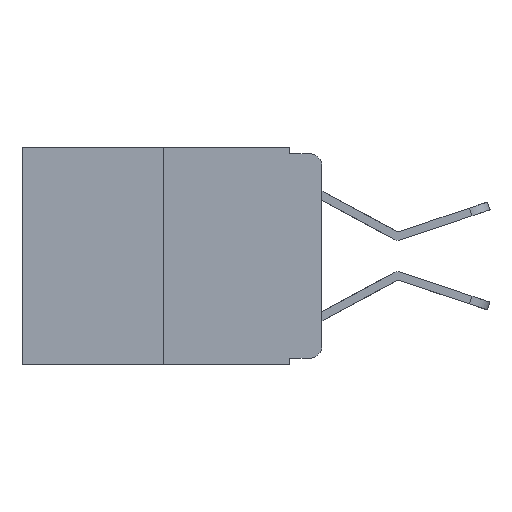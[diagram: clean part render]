
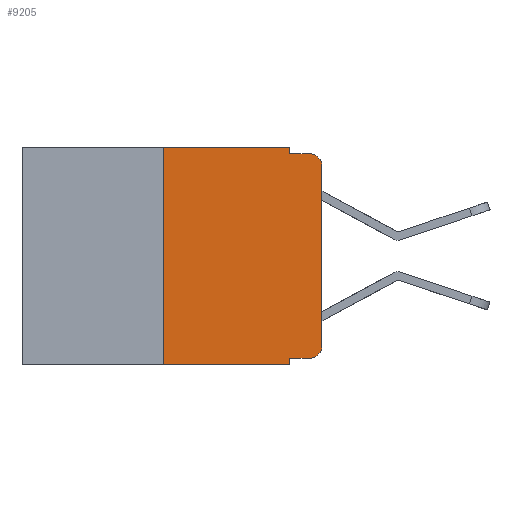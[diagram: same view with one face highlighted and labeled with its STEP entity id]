
A CAD part, left-side view. The second image highlights one B-rep face of the part: STEP entity #9205.
In plain terms, the highlighted planar face has unit normal (-1, 0, 0).
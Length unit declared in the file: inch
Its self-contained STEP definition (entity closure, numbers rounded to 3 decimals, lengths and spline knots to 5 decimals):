
#438 = CARTESIAN_POINT ( 'NONE',  ( 0., 0.051, -0.343 ) ) ;
#511 = DIRECTION ( 'NONE',  ( 0., 0., 1. ) ) ;
#538 = CARTESIAN_POINT ( 'NONE',  ( 0., 0., -0.03 ) ) ;
#571 = VERTEX_POINT ( 'NONE', #6471 ) ;
#1121 = VERTEX_POINT ( 'NONE', #14842 ) ;
#1142 = DIRECTION ( 'NONE',  ( 0., -1., 0. ) ) ;
#1658 = EDGE_CURVE ( 'NONE', #22719, #10213, #4527, .T. ) ;
#1781 = CARTESIAN_POINT ( 'NONE',  ( 0., 0.051, -0.333 ) ) ;
#1842 = DIRECTION ( 'NONE',  ( 1., 0., 0. ) ) ;
#2128 = EDGE_CURVE ( 'NONE', #10508, #6056, #24708, .T. ) ;
#3127 = ORIENTED_EDGE ( 'NONE', *, *, #15322, .T. ) ;
#3348 = DIRECTION ( 'NONE',  ( 0., -1., 0. ) ) ;
#3583 = ORIENTED_EDGE ( 'NONE', *, *, #8295, .F. ) ;
#4527 = CIRCLE ( 'NONE', #18561, 0.02 ) ;
#5476 = CARTESIAN_POINT ( 'NONE',  ( 0., 0., -0.313 ) ) ;
#5911 = DIRECTION ( 'NONE',  ( 0., -1., 0. ) ) ;
#6002 = LINE ( 'NONE', #9131, #11270 ) ;
#6056 = VERTEX_POINT ( 'NONE', #16016 ) ;
#6241 = VECTOR ( 'NONE', #3348, 39.37008 ) ;
#6471 = CARTESIAN_POINT ( 'NONE',  ( 0., 0.051, -0.333 ) ) ;
#6714 = ORIENTED_EDGE ( 'NONE', *, *, #10706, .T. ) ;
#7029 = CARTESIAN_POINT ( 'NONE',  ( 0., 0.051, -0.01 ) ) ;
#7503 = CARTESIAN_POINT ( 'NONE',  ( 0., 0.051, 0. ) ) ;
#7619 = DIRECTION ( 'NONE',  ( -1., 0., 0. ) ) ;
#7758 = CARTESIAN_POINT ( 'NONE',  ( 0., 0.02, -0.313 ) ) ;
#8006 = ORIENTED_EDGE ( 'NONE', *, *, #16729, .T. ) ;
#8295 = EDGE_CURVE ( 'NONE', #25612, #6056, #15109, .T. ) ;
#8587 = CARTESIAN_POINT ( 'NONE',  ( 0., 0.473, -0.343 ) ) ;
#8713 = VECTOR ( 'NONE', #17361, 39.37008 ) ;
#9131 = CARTESIAN_POINT ( 'NONE',  ( 0., 0.051, 0. ) ) ;
#9184 = LINE ( 'NONE', #1781, #18407 ) ;
#9205 = ADVANCED_FACE ( 'NONE', ( #10983 ), #17691, .F. ) ;
#9241 = LINE ( 'NONE', #16446, #24197 ) ;
#9518 = EDGE_LOOP ( 'NONE', ( #6714, #20879, #3583, #24543, #12694, #20424, #3127, #12932, #8006, #22412 ) ) ;
#9790 = DIRECTION ( 'NONE',  ( 0., 0., -1. ) ) ;
#9868 = CARTESIAN_POINT ( 'NONE',  ( 0., 0.473, 0. ) ) ;
#9884 = LINE ( 'NONE', #8587, #20317 ) ;
#9987 = CARTESIAN_POINT ( 'NONE',  ( 0., 0.25, 0. ) ) ;
#10110 = EDGE_CURVE ( 'NONE', #1121, #25612, #6002, .T. ) ;
#10213 = VERTEX_POINT ( 'NONE', #5476 ) ;
#10508 = VERTEX_POINT ( 'NONE', #538 ) ;
#10706 = EDGE_CURVE ( 'NONE', #10213, #10508, #23738, .T. ) ;
#10983 = FACE_OUTER_BOUND ( 'NONE', #9518, .T. ) ;
#11186 = EDGE_CURVE ( 'NONE', #14637, #1121, #12133, .T. ) ;
#11270 = VECTOR ( 'NONE', #22784, 39.37008 ) ;
#12133 = LINE ( 'NONE', #24802, #6241 ) ;
#12478 = DIRECTION ( 'NONE',  ( 0., -1., 0. ) ) ;
#12694 = ORIENTED_EDGE ( 'NONE', *, *, #11186, .F. ) ;
#12905 = EDGE_CURVE ( 'NONE', #17316, #14637, #9241, .T. ) ;
#12932 = ORIENTED_EDGE ( 'NONE', *, *, #21120, .F. ) ;
#14637 = VERTEX_POINT ( 'NONE', #9987 ) ;
#14842 = CARTESIAN_POINT ( 'NONE',  ( 0., 0.051, 0. ) ) ;
#15107 = CARTESIAN_POINT ( 'NONE',  ( 0., 0.051, -0.01 ) ) ;
#15109 = LINE ( 'NONE', #15107, #18522 ) ;
#15322 = EDGE_CURVE ( 'NONE', #17316, #24985, #9884, .T. ) ;
#15768 = DIRECTION ( 'NONE',  ( 0., 0., -1. ) ) ;
#16016 = CARTESIAN_POINT ( 'NONE',  ( 0., 0.02, -0.01 ) ) ;
#16446 = CARTESIAN_POINT ( 'NONE',  ( 0., 0.25, 0. ) ) ;
#16729 = EDGE_CURVE ( 'NONE', #571, #22719, #9184, .T. ) ;
#17316 = VERTEX_POINT ( 'NONE', #21346 ) ;
#17361 = DIRECTION ( 'NONE',  ( 0., 0., -1. ) ) ;
#17691 = PLANE ( 'NONE',  #25461 ) ;
#18407 = VECTOR ( 'NONE', #5911, 39.37008 ) ;
#18522 = VECTOR ( 'NONE', #1142, 39.37008 ) ;
#18561 = AXIS2_PLACEMENT_3D ( 'NONE', #7758, #21504, #9790 ) ;
#19155 = LINE ( 'NONE', #7503, #8713 ) ;
#19410 = CARTESIAN_POINT ( 'NONE',  ( 0., 0.02, -0.03 ) ) ;
#20317 = VECTOR ( 'NONE', #12478, 39.37008 ) ;
#20424 = ORIENTED_EDGE ( 'NONE', *, *, #12905, .F. ) ;
#20879 = ORIENTED_EDGE ( 'NONE', *, *, #2128, .T. ) ;
#21083 = DIRECTION ( 'NONE',  ( 0., 0., 1. ) ) ;
#21120 = EDGE_CURVE ( 'NONE', #571, #24985, #19155, .T. ) ;
#21277 = CARTESIAN_POINT ( 'NONE',  ( 0., 0.02, -0.333 ) ) ;
#21346 = CARTESIAN_POINT ( 'NONE',  ( 0., 0.25, -0.343 ) ) ;
#21381 = DIRECTION ( 'NONE',  ( 0., 0., -1. ) ) ;
#21504 = DIRECTION ( 'NONE',  ( -1., 0., 0. ) ) ;
#21961 = AXIS2_PLACEMENT_3D ( 'NONE', #19410, #7619, #21381 ) ;
#22412 = ORIENTED_EDGE ( 'NONE', *, *, #1658, .T. ) ;
#22719 = VERTEX_POINT ( 'NONE', #21277 ) ;
#22784 = DIRECTION ( 'NONE',  ( 0., 0., -1. ) ) ;
#22908 = CARTESIAN_POINT ( 'NONE',  ( 0., 0., 0. ) ) ;
#23124 = VECTOR ( 'NONE', #21083, 39.37008 ) ;
#23738 = LINE ( 'NONE', #22908, #23124 ) ;
#24197 = VECTOR ( 'NONE', #511, 39.37008 ) ;
#24543 = ORIENTED_EDGE ( 'NONE', *, *, #10110, .F. ) ;
#24708 = CIRCLE ( 'NONE', #21961, 0.02 ) ;
#24802 = CARTESIAN_POINT ( 'NONE',  ( 0., 0.473, 0. ) ) ;
#24985 = VERTEX_POINT ( 'NONE', #438 ) ;
#25461 = AXIS2_PLACEMENT_3D ( 'NONE', #9868, #1842, #15768 ) ;
#25612 = VERTEX_POINT ( 'NONE', #7029 ) ;
